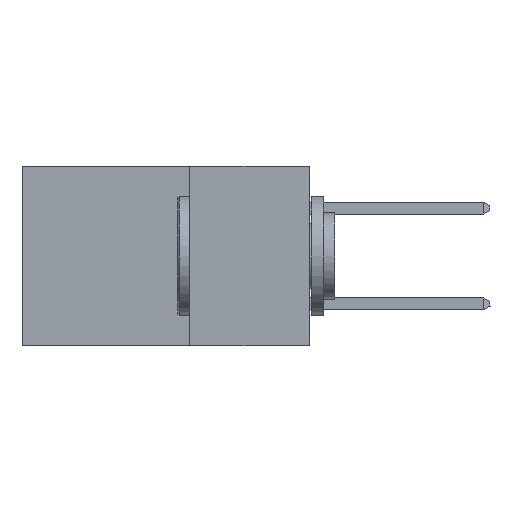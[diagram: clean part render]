
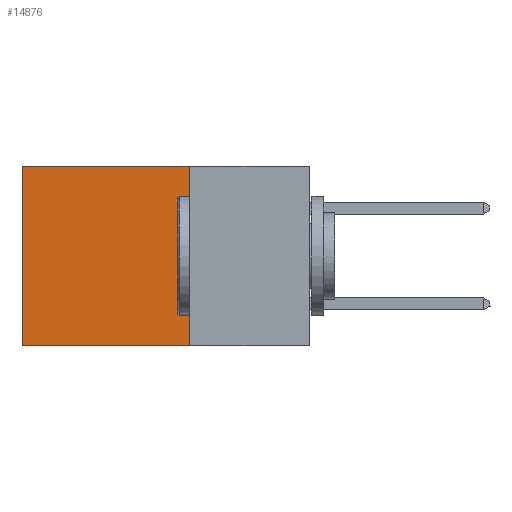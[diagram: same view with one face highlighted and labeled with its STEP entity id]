
A CAD part, left-side view. The second image highlights one B-rep face of the part: STEP entity #14876.
In plain terms, the highlighted planar face has unit normal (-1, 0, 0).
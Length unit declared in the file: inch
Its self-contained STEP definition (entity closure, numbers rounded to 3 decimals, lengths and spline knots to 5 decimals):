
#108 = VERTEX_POINT ( 'NONE', #9827 ) ;
#598 = CARTESIAN_POINT ( 'NONE',  ( 0.2875, 0.25, -0.375 ) ) ;
#2440 = VECTOR ( 'NONE', #8480, 39.37008 ) ;
#3306 = EDGE_CURVE ( 'NONE', #15121, #6839, #9128, .T. ) ;
#3485 = EDGE_CURVE ( 'NONE', #15121, #108, #13264, .T. ) ;
#3606 = CARTESIAN_POINT ( 'NONE',  ( 0.2875, 0.25, -0.375 ) ) ;
#3874 = VECTOR ( 'NONE', #6381, 39.37008 ) ;
#4378 = CARTESIAN_POINT ( 'NONE',  ( 0.2875, 0.6, -0.375 ) ) ;
#4415 = ORIENTED_EDGE ( 'NONE', *, *, #11550, .F. ) ;
#4575 = CARTESIAN_POINT ( 'NONE',  ( 0.2875, 0.25, -0.375 ) ) ;
#4632 = CARTESIAN_POINT ( 'NONE',  ( 0.2875, 0.25, 0. ) ) ;
#5000 = CARTESIAN_POINT ( 'NONE',  ( 0.2875, 0.25, 0. ) ) ;
#5619 = LINE ( 'NONE', #9625, #2440 ) ;
#5784 = ORIENTED_EDGE ( 'NONE', *, *, #3306, .F. ) ;
#5999 = VERTEX_POINT ( 'NONE', #4378 ) ;
#6381 = DIRECTION ( 'NONE',  ( 0., 1., 0. ) ) ;
#6839 = VERTEX_POINT ( 'NONE', #4575 ) ;
#7682 = EDGE_LOOP ( 'NONE', ( #16305, #4415, #5784, #11676 ) ) ;
#8128 = VECTOR ( 'NONE', #13483, 39.37008 ) ;
#8136 = AXIS2_PLACEMENT_3D ( 'NONE', #3606, #13671, #8552 ) ;
#8480 = DIRECTION ( 'NONE',  ( 0., 0., -1. ) ) ;
#8552 = DIRECTION ( 'NONE',  ( 0., 0., -1. ) ) ;
#9128 = LINE ( 'NONE', #598, #15455 ) ;
#9625 = CARTESIAN_POINT ( 'NONE',  ( 0.2875, 0.6, -0.375 ) ) ;
#9801 = CARTESIAN_POINT ( 'NONE',  ( 0.2875, 0.25, -0.375 ) ) ;
#9827 = CARTESIAN_POINT ( 'NONE',  ( 0.2875, 0.6, 0. ) ) ;
#10729 = DIRECTION ( 'NONE',  ( 0., 0., -1. ) ) ;
#11550 = EDGE_CURVE ( 'NONE', #6839, #5999, #15748, .T. ) ;
#11676 = ORIENTED_EDGE ( 'NONE', *, *, #3485, .T. ) ;
#12191 = EDGE_CURVE ( 'NONE', #108, #5999, #5619, .T. ) ;
#13264 = LINE ( 'NONE', #4632, #8128 ) ;
#13483 = DIRECTION ( 'NONE',  ( 0., 1., 0. ) ) ;
#13671 = DIRECTION ( 'NONE',  ( 1., 0., 0. ) ) ;
#14497 = FACE_OUTER_BOUND ( 'NONE', #7682, .T. ) ;
#14876 = ADVANCED_FACE ( 'NONE', ( #14497 ), #16300, .F. ) ;
#15121 = VERTEX_POINT ( 'NONE', #5000 ) ;
#15455 = VECTOR ( 'NONE', #10729, 39.37008 ) ;
#15748 = LINE ( 'NONE', #9801, #3874 ) ;
#16300 = PLANE ( 'NONE',  #8136 ) ;
#16305 = ORIENTED_EDGE ( 'NONE', *, *, #12191, .T. ) ;
